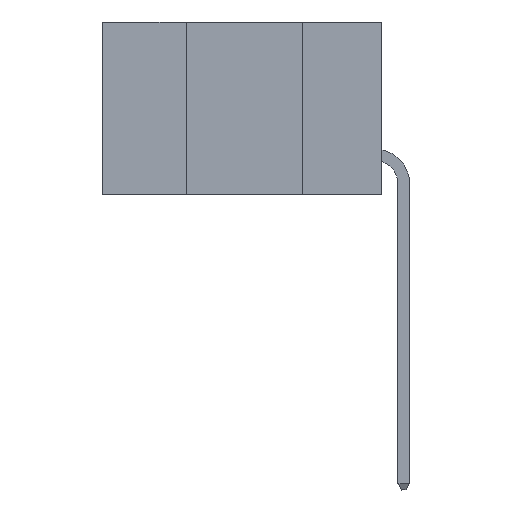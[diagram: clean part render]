
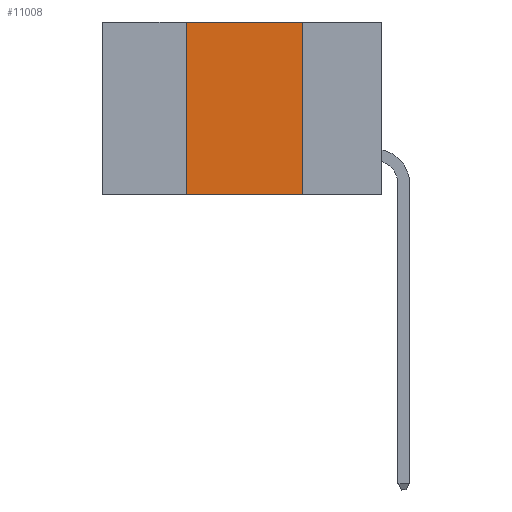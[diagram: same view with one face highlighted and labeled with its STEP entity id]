
A CAD part, left-side view. The second image highlights one B-rep face of the part: STEP entity #11008.
In plain terms, the highlighted planar face has unit normal (-1, 0, 0).
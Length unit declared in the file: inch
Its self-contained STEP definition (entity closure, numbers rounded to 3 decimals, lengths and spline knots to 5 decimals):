
#1067 = DIRECTION ( 'NONE',  ( 0., -1., 0. ) ) ;
#1770 = VERTEX_POINT ( 'NONE', #18973 ) ;
#3158 = CARTESIAN_POINT ( 'NONE',  ( 0., 0.6, -0.37 ) ) ;
#4716 = LINE ( 'NONE', #23241, #37692 ) ;
#4887 = CARTESIAN_POINT ( 'NONE',  ( 0., 0.17, 0. ) ) ;
#5213 = EDGE_CURVE ( 'NONE', #18562, #8878, #4716, .T. ) ;
#5347 = EDGE_LOOP ( 'NONE', ( #44562, #31279, #17815, #32902 ) ) ;
#7834 = PLANE ( 'NONE',  #44413 ) ;
#8878 = VERTEX_POINT ( 'NONE', #10798 ) ;
#9168 = DIRECTION ( 'NONE',  ( 0., -1., 0. ) ) ;
#10798 = CARTESIAN_POINT ( 'NONE',  ( 0., 0.17, 0. ) ) ;
#10801 = EDGE_CURVE ( 'NONE', #32553, #1770, #40304, .T. ) ;
#11008 = ADVANCED_FACE ( 'NONE', ( #11526 ), #7834, .F. ) ;
#11526 = FACE_OUTER_BOUND ( 'NONE', #5347, .T. ) ;
#12164 = CARTESIAN_POINT ( 'NONE',  ( 0., 0.42, -0.37 ) ) ;
#16537 = VECTOR ( 'NONE', #39932, 39.37008 ) ;
#17815 = ORIENTED_EDGE ( 'NONE', *, *, #29456, .F. ) ;
#18216 = DIRECTION ( 'NONE',  ( 0., 0., -1. ) ) ;
#18222 = DIRECTION ( 'NONE',  ( 0., 0., -1. ) ) ;
#18562 = VERTEX_POINT ( 'NONE', #42052 ) ;
#18973 = CARTESIAN_POINT ( 'NONE',  ( 0., 0.17, -0.37 ) ) ;
#23241 = CARTESIAN_POINT ( 'NONE',  ( 0., 0.6, 0. ) ) ;
#27340 = CARTESIAN_POINT ( 'NONE',  ( 0., 0.6, 0. ) ) ;
#28873 = CARTESIAN_POINT ( 'NONE',  ( 0., 0.42, 0. ) ) ;
#29456 = EDGE_CURVE ( 'NONE', #32553, #18562, #37103, .T. ) ;
#31091 = VECTOR ( 'NONE', #1067, 39.37008 ) ;
#31279 = ORIENTED_EDGE ( 'NONE', *, *, #5213, .F. ) ;
#32553 = VERTEX_POINT ( 'NONE', #12164 ) ;
#32902 = ORIENTED_EDGE ( 'NONE', *, *, #10801, .T. ) ;
#34289 = LINE ( 'NONE', #4887, #40214 ) ;
#37103 = LINE ( 'NONE', #28873, #16537 ) ;
#37692 = VECTOR ( 'NONE', #9168, 39.37008 ) ;
#38665 = DIRECTION ( 'NONE',  ( 1., 0., 0. ) ) ;
#39932 = DIRECTION ( 'NONE',  ( 0., 0., 1. ) ) ;
#40214 = VECTOR ( 'NONE', #18216, 39.37008 ) ;
#40304 = LINE ( 'NONE', #3158, #31091 ) ;
#40716 = EDGE_CURVE ( 'NONE', #8878, #1770, #34289, .T. ) ;
#42052 = CARTESIAN_POINT ( 'NONE',  ( 0., 0.42, 0. ) ) ;
#44413 = AXIS2_PLACEMENT_3D ( 'NONE', #27340, #38665, #18222 ) ;
#44562 = ORIENTED_EDGE ( 'NONE', *, *, #40716, .F. ) ;
